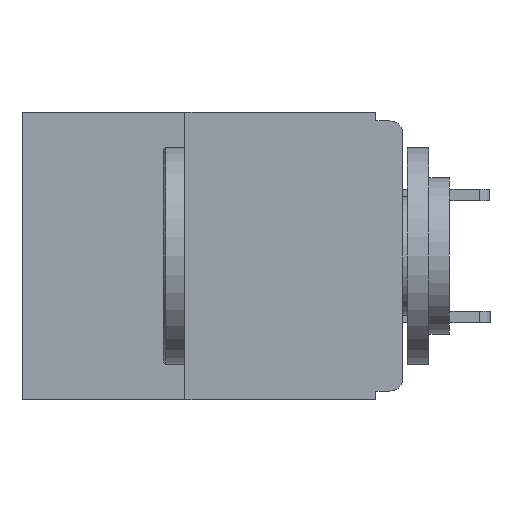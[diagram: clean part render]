
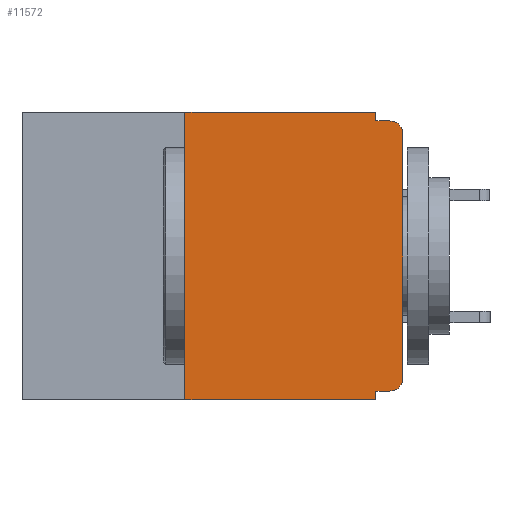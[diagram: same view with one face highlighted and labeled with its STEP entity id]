
A CAD part, left-side view. The second image highlights one B-rep face of the part: STEP entity #11572.
In plain terms, the highlighted planar face has unit normal (-1, 0, 0).
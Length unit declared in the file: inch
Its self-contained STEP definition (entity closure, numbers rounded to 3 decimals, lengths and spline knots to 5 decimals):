
#981 = CARTESIAN_POINT ( 'NONE',  ( 0., 0.437, 0. ) ) ;
#1044 = VERTEX_POINT ( 'NONE', #10934 ) ;
#1128 = CARTESIAN_POINT ( 'NONE',  ( 0., 0.25, -0.33 ) ) ;
#1157 = EDGE_CURVE ( 'NONE', #11734, #5712, #4671, .T. ) ;
#1351 = VERTEX_POINT ( 'NONE', #12238 ) ;
#1579 = ORIENTED_EDGE ( 'NONE', *, *, #5561, .T. ) ;
#1611 = VECTOR ( 'NONE', #12885, 39.37008 ) ;
#1659 = LINE ( 'NONE', #11376, #12905 ) ;
#1715 = EDGE_CURVE ( 'NONE', #1351, #4855, #8401, .T. ) ;
#1986 = DIRECTION ( 'NONE',  ( 0., 0., -1. ) ) ;
#2073 = LINE ( 'NONE', #981, #13605 ) ;
#2220 = VECTOR ( 'NONE', #8447, 39.37008 ) ;
#2653 = EDGE_CURVE ( 'NONE', #14203, #5783, #8030, .T. ) ;
#3403 = EDGE_CURVE ( 'NONE', #7080, #5100, #13213, .T. ) ;
#3640 = FACE_OUTER_BOUND ( 'NONE', #8803, .T. ) ;
#4289 = AXIS2_PLACEMENT_3D ( 'NONE', #6350, #8578, #1986 ) ;
#4671 = CIRCLE ( 'NONE', #7021, 0.015 ) ;
#4855 = VERTEX_POINT ( 'NONE', #8679 ) ;
#5100 = VERTEX_POINT ( 'NONE', #5248 ) ;
#5150 = VECTOR ( 'NONE', #12773, 39.37008 ) ;
#5151 = VECTOR ( 'NONE', #6413, 39.37008 ) ;
#5248 = CARTESIAN_POINT ( 'NONE',  ( 0., 0.25, 0. ) ) ;
#5315 = CARTESIAN_POINT ( 'NONE',  ( 0., 0.031, 0. ) ) ;
#5561 = EDGE_CURVE ( 'NONE', #1044, #12253, #5589, .T. ) ;
#5582 = CARTESIAN_POINT ( 'NONE',  ( 0., 0.015, -0.01 ) ) ;
#5589 = CIRCLE ( 'NONE', #5915, 0.015 ) ;
#5640 = DIRECTION ( 'NONE',  ( -1., 0., 0. ) ) ;
#5712 = VERTEX_POINT ( 'NONE', #11515 ) ;
#5759 = EDGE_CURVE ( 'NONE', #7080, #5783, #1659, .T. ) ;
#5783 = VERTEX_POINT ( 'NONE', #10977 ) ;
#5827 = DIRECTION ( 'NONE',  ( 0., 0., -1. ) ) ;
#5849 = ORIENTED_EDGE ( 'NONE', *, *, #1715, .F. ) ;
#5915 = AXIS2_PLACEMENT_3D ( 'NONE', #12671, #12648, #12635 ) ;
#6017 = ORIENTED_EDGE ( 'NONE', *, *, #11054, .F. ) ;
#6179 = EDGE_CURVE ( 'NONE', #4855, #12253, #13560, .T. ) ;
#6256 = CARTESIAN_POINT ( 'NONE',  ( 0., 0., -0.32 ) ) ;
#6350 = CARTESIAN_POINT ( 'NONE',  ( 0., 0.437, 0. ) ) ;
#6397 = PLANE ( 'NONE',  #4289 ) ;
#6413 = DIRECTION ( 'NONE',  ( 0., 1., 0. ) ) ;
#6414 = EDGE_CURVE ( 'NONE', #11734, #14203, #13718, .T. ) ;
#6468 = ORIENTED_EDGE ( 'NONE', *, *, #7538, .T. ) ;
#7021 = AXIS2_PLACEMENT_3D ( 'NONE', #10877, #5640, #5827 ) ;
#7080 = VERTEX_POINT ( 'NONE', #1128 ) ;
#7309 = ORIENTED_EDGE ( 'NONE', *, *, #1157, .T. ) ;
#7538 = EDGE_CURVE ( 'NONE', #5712, #1044, #13854, .T. ) ;
#7632 = DIRECTION ( 'NONE',  ( 0., -1., 0. ) ) ;
#7634 = DIRECTION ( 'NONE',  ( 0., 0., 1. ) ) ;
#7798 = ORIENTED_EDGE ( 'NONE', *, *, #6414, .F. ) ;
#8030 = LINE ( 'NONE', #10788, #5150 ) ;
#8107 = CARTESIAN_POINT ( 'NONE',  ( 0., 0.031, -0.32 ) ) ;
#8209 = DIRECTION ( 'NONE',  ( 0., -1., 0. ) ) ;
#8238 = CARTESIAN_POINT ( 'NONE',  ( 0., 0., -0.01 ) ) ;
#8401 = LINE ( 'NONE', #5315, #2220 ) ;
#8447 = DIRECTION ( 'NONE',  ( 0., 0., -1. ) ) ;
#8578 = DIRECTION ( 'NONE',  ( 1., 0., 0. ) ) ;
#8679 = CARTESIAN_POINT ( 'NONE',  ( 0., 0.031, -0.01 ) ) ;
#8803 = EDGE_LOOP ( 'NONE', ( #6468, #1579, #12001, #5849, #6017, #9064, #9396, #9571, #7798, #7309 ) ) ;
#9064 = ORIENTED_EDGE ( 'NONE', *, *, #3403, .F. ) ;
#9396 = ORIENTED_EDGE ( 'NONE', *, *, #5759, .T. ) ;
#9571 = ORIENTED_EDGE ( 'NONE', *, *, #2653, .F. ) ;
#10705 = VECTOR ( 'NONE', #8209, 39.37008 ) ;
#10788 = CARTESIAN_POINT ( 'NONE',  ( 0., 0.031, -0.33 ) ) ;
#10877 = CARTESIAN_POINT ( 'NONE',  ( 0., 0.015, -0.305 ) ) ;
#10934 = CARTESIAN_POINT ( 'NONE',  ( 0., 0., -0.025 ) ) ;
#10977 = CARTESIAN_POINT ( 'NONE',  ( 0., 0.031, -0.33 ) ) ;
#11054 = EDGE_CURVE ( 'NONE', #5100, #1351, #2073, .T. ) ;
#11110 = CARTESIAN_POINT ( 'NONE',  ( 0., 0.015, -0.32 ) ) ;
#11145 = DIRECTION ( 'NONE',  ( 0., -1., 0. ) ) ;
#11376 = CARTESIAN_POINT ( 'NONE',  ( 0., 0.437, -0.33 ) ) ;
#11515 = CARTESIAN_POINT ( 'NONE',  ( 0., 0., -0.305 ) ) ;
#11572 = ADVANCED_FACE ( 'NONE', ( #3640 ), #6397, .F. ) ;
#11734 = VERTEX_POINT ( 'NONE', #11110 ) ;
#11876 = CARTESIAN_POINT ( 'NONE',  ( 0., 0., 0. ) ) ;
#12001 = ORIENTED_EDGE ( 'NONE', *, *, #6179, .F. ) ;
#12169 = CARTESIAN_POINT ( 'NONE',  ( 0., 0.25, -0.33 ) ) ;
#12238 = CARTESIAN_POINT ( 'NONE',  ( 0., 0.031, 0. ) ) ;
#12253 = VERTEX_POINT ( 'NONE', #5582 ) ;
#12635 = DIRECTION ( 'NONE',  ( 0., 0., -1. ) ) ;
#12648 = DIRECTION ( 'NONE',  ( -1., 0., 0. ) ) ;
#12671 = CARTESIAN_POINT ( 'NONE',  ( 0., 0.015, -0.025 ) ) ;
#12773 = DIRECTION ( 'NONE',  ( 0., 0., -1. ) ) ;
#12885 = DIRECTION ( 'NONE',  ( 0., 0., 1. ) ) ;
#12905 = VECTOR ( 'NONE', #11145, 39.37008 ) ;
#13213 = LINE ( 'NONE', #12169, #1611 ) ;
#13528 = VECTOR ( 'NONE', #7634, 39.37008 ) ;
#13560 = LINE ( 'NONE', #8238, #10705 ) ;
#13605 = VECTOR ( 'NONE', #7632, 39.37008 ) ;
#13718 = LINE ( 'NONE', #6256, #5151 ) ;
#13854 = LINE ( 'NONE', #11876, #13528 ) ;
#14203 = VERTEX_POINT ( 'NONE', #8107 ) ;
